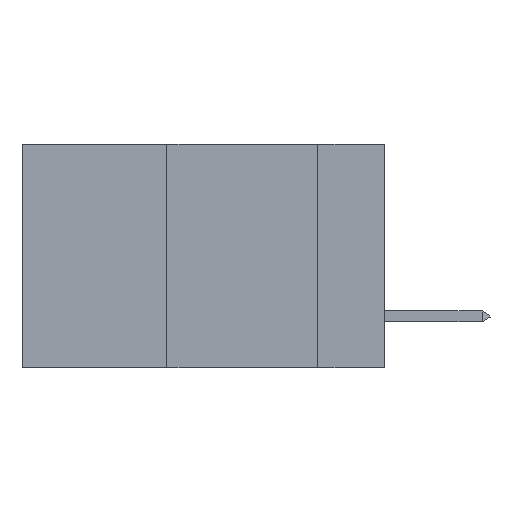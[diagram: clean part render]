
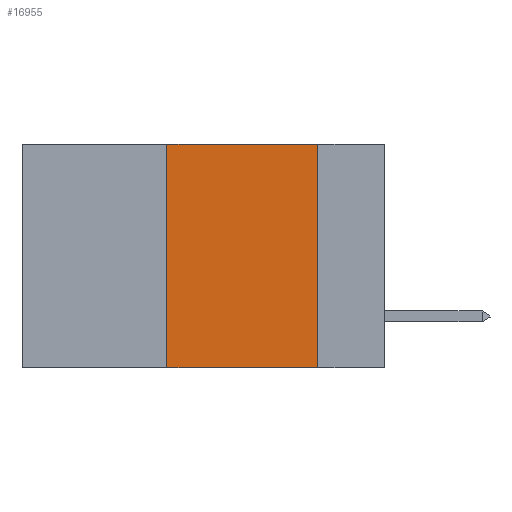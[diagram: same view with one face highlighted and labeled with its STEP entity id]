
A CAD part, left-side view. The second image highlights one B-rep face of the part: STEP entity #16955.
In plain terms, the highlighted planar face has unit normal (-1, 0, 0).
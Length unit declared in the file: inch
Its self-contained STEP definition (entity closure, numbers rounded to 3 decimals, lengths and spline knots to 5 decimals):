
#922 = ORIENTED_EDGE ( 'NONE', *, *, #8687, .F. ) ;
#1026 = VERTEX_POINT ( 'NONE', #12567 ) ;
#2268 = ORIENTED_EDGE ( 'NONE', *, *, #21997, .T. ) ;
#2304 = DIRECTION ( 'NONE',  ( 0., -1., 0. ) ) ;
#2528 = CARTESIAN_POINT ( 'NONE',  ( 0., 0.6, 0. ) ) ;
#3914 = VECTOR ( 'NONE', #17880, 39.37008 ) ;
#4305 = DIRECTION ( 'NONE',  ( 0., 0., -1. ) ) ;
#4961 = DIRECTION ( 'NONE',  ( 0., 0., 1. ) ) ;
#5037 = ORIENTED_EDGE ( 'NONE', *, *, #19503, .F. ) ;
#5041 = VECTOR ( 'NONE', #4961, 39.37008 ) ;
#5096 = EDGE_LOOP ( 'NONE', ( #922, #5037, #18226, #2268 ) ) ;
#7090 = VERTEX_POINT ( 'NONE', #9116 ) ;
#7422 = LINE ( 'NONE', #19696, #3914 ) ;
#7542 = LINE ( 'NONE', #2528, #18104 ) ;
#7760 = VERTEX_POINT ( 'NONE', #16292 ) ;
#7901 = CARTESIAN_POINT ( 'NONE',  ( 0., 0.6, 0. ) ) ;
#8608 = VECTOR ( 'NONE', #13786, 39.37008 ) ;
#8687 = EDGE_CURVE ( 'NONE', #22443, #7090, #17417, .T. ) ;
#9116 = CARTESIAN_POINT ( 'NONE',  ( 0., 0.11, -0.37 ) ) ;
#12567 = CARTESIAN_POINT ( 'NONE',  ( 0., 0.36, -0.37 ) ) ;
#13624 = CARTESIAN_POINT ( 'NONE',  ( 0., 0.11, 0. ) ) ;
#13726 = DIRECTION ( 'NONE',  ( 1., 0., 0. ) ) ;
#13786 = DIRECTION ( 'NONE',  ( 0., 0., -1. ) ) ;
#13861 = CARTESIAN_POINT ( 'NONE',  ( 0., 0.11, 0. ) ) ;
#14727 = FACE_OUTER_BOUND ( 'NONE', #5096, .T. ) ;
#15038 = LINE ( 'NONE', #23806, #5041 ) ;
#15475 = PLANE ( 'NONE',  #17442 ) ;
#16292 = CARTESIAN_POINT ( 'NONE',  ( 0., 0.36, 0. ) ) ;
#16955 = ADVANCED_FACE ( 'NONE', ( #14727 ), #15475, .F. ) ;
#17417 = LINE ( 'NONE', #13861, #8608 ) ;
#17442 = AXIS2_PLACEMENT_3D ( 'NONE', #7901, #13726, #4305 ) ;
#17880 = DIRECTION ( 'NONE',  ( 0., -1., 0. ) ) ;
#18104 = VECTOR ( 'NONE', #2304, 39.37008 ) ;
#18226 = ORIENTED_EDGE ( 'NONE', *, *, #23352, .F. ) ;
#19503 = EDGE_CURVE ( 'NONE', #7760, #22443, #7542, .T. ) ;
#19696 = CARTESIAN_POINT ( 'NONE',  ( 0., 0.6, -0.37 ) ) ;
#21997 = EDGE_CURVE ( 'NONE', #1026, #7090, #7422, .T. ) ;
#22443 = VERTEX_POINT ( 'NONE', #13624 ) ;
#23352 = EDGE_CURVE ( 'NONE', #1026, #7760, #15038, .T. ) ;
#23806 = CARTESIAN_POINT ( 'NONE',  ( 0., 0.36, 0. ) ) ;
